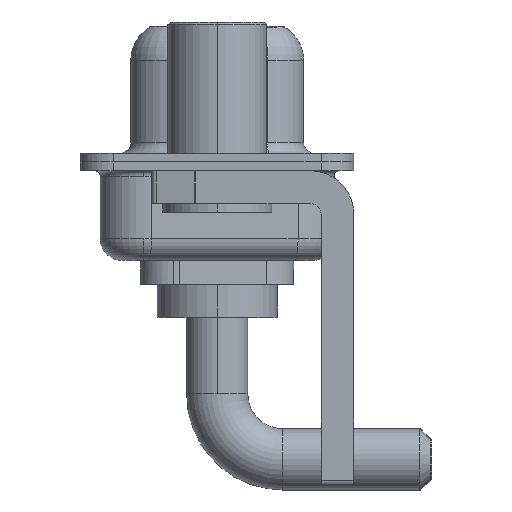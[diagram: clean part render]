
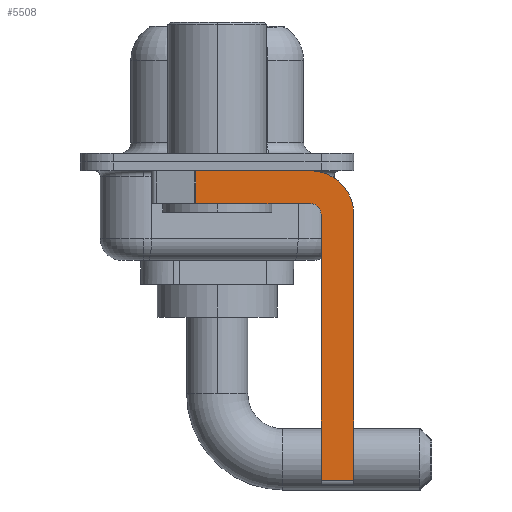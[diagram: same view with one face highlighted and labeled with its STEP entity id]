
A CAD part, left-side view. The second image highlights one B-rep face of the part: STEP entity #5508.
In plain terms, the highlighted planar face has unit normal (-1, 0, 0).
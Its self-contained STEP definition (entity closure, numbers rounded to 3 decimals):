
#677 = LINE ( 'NONE', #7979, #12336 ) ;
#777 = LINE ( 'NONE', #11700, #1538 ) ;
#812 = EDGE_CURVE ( 'NONE', #5361, #9923, #4847, .T. ) ;
#1538 = VECTOR ( 'NONE', #4550, 1000. ) ;
#1557 = AXIS2_PLACEMENT_3D ( 'NONE', #3761, #6102, #3675 ) ;
#2128 = VERTEX_POINT ( 'NONE', #10111 ) ;
#2206 = CARTESIAN_POINT ( 'NONE',  ( -2.9, 3., -0.4 ) ) ;
#2363 = CARTESIAN_POINT ( 'NONE',  ( -2.9, -4.25, -1.9 ) ) ;
#2374 = ORIENTED_EDGE ( 'NONE', *, *, #7991, .F. ) ;
#2444 = LINE ( 'NONE', #2363, #6817 ) ;
#2499 = AXIS2_PLACEMENT_3D ( 'NONE', #13245, #7312, #13542 ) ;
#2978 = VERTEX_POINT ( 'NONE', #5662 ) ;
#3033 = EDGE_CURVE ( 'NONE', #4386, #2978, #11764, .T. ) ;
#3071 = LINE ( 'NONE', #9015, #6953 ) ;
#3115 = CIRCLE ( 'NONE', #6193, 0.5 ) ;
#3116 = DIRECTION ( 'NONE',  ( -1., 0., 0. ) ) ;
#3157 = EDGE_CURVE ( 'NONE', #14407, #2128, #2444, .T. ) ;
#3183 = DIRECTION ( 'NONE',  ( 0., -1., 0. ) ) ;
#3310 = ORIENTED_EDGE ( 'NONE', *, *, #11388, .F. ) ;
#3675 = DIRECTION ( 'NONE',  ( 0., 0., -1. ) ) ;
#3761 = CARTESIAN_POINT ( 'NONE',  ( -2.9, -4.25, -2.4 ) ) ;
#3883 = CARTESIAN_POINT ( 'NONE',  ( -2.9, -4.25, -14.55 ) ) ;
#4066 = ORIENTED_EDGE ( 'NONE', *, *, #15296, .F. ) ;
#4386 = VERTEX_POINT ( 'NONE', #14305 ) ;
#4550 = DIRECTION ( 'NONE',  ( 0., 0., -1. ) ) ;
#4676 = CARTESIAN_POINT ( 'NONE',  ( -2.9, -4.25, -1.9 ) ) ;
#4727 = EDGE_LOOP ( 'NONE', ( #10317, #12907, #7708, #7586, #3310, #14551, #4066, #2374 ) ) ;
#4847 = LINE ( 'NONE', #3883, #8808 ) ;
#5361 = VERTEX_POINT ( 'NONE', #13079 ) ;
#5508 = ADVANCED_FACE ( 'NONE', ( #13474 ), #8686, .F. ) ;
#5662 = CARTESIAN_POINT ( 'NONE',  ( -2.9, -4.25, -0.4 ) ) ;
#5808 = CARTESIAN_POINT ( 'NONE',  ( -2.9, -6.25, -2.4 ) ) ;
#6102 = DIRECTION ( 'NONE',  ( 1., 0., 0. ) ) ;
#6193 = AXIS2_PLACEMENT_3D ( 'NONE', #15276, #3116, #14318 ) ;
#6817 = VECTOR ( 'NONE', #15815, 1000. ) ;
#6953 = VECTOR ( 'NONE', #15230, 1000. ) ;
#6992 = EDGE_CURVE ( 'NONE', #4386, #2128, #3071, .T. ) ;
#7120 = VERTEX_POINT ( 'NONE', #7720 ) ;
#7312 = DIRECTION ( 'NONE',  ( 1., 0., 0. ) ) ;
#7586 = ORIENTED_EDGE ( 'NONE', *, *, #9136, .F. ) ;
#7708 = ORIENTED_EDGE ( 'NONE', *, *, #3157, .F. ) ;
#7720 = CARTESIAN_POINT ( 'NONE',  ( -2.9, -4.75, -2.4 ) ) ;
#7979 = CARTESIAN_POINT ( 'NONE',  ( -2.9, -4.75, -14.8 ) ) ;
#7991 = EDGE_CURVE ( 'NONE', #2978, #8570, #12068, .T. ) ;
#8570 = VERTEX_POINT ( 'NONE', #5808 ) ;
#8686 = PLANE ( 'NONE',  #2499 ) ;
#8808 = VECTOR ( 'NONE', #14842, 1000. ) ;
#9015 = CARTESIAN_POINT ( 'NONE',  ( -2.9, 0.978, -1.9 ) ) ;
#9110 = CARTESIAN_POINT ( 'NONE',  ( -2.9, -6.25, -14.55 ) ) ;
#9136 = EDGE_CURVE ( 'NONE', #7120, #14407, #3115, .T. ) ;
#9923 = VERTEX_POINT ( 'NONE', #9110 ) ;
#10111 = CARTESIAN_POINT ( 'NONE',  ( -2.9, 0.978, -1.9 ) ) ;
#10317 = ORIENTED_EDGE ( 'NONE', *, *, #3033, .F. ) ;
#11388 = EDGE_CURVE ( 'NONE', #5361, #7120, #677, .T. ) ;
#11700 = CARTESIAN_POINT ( 'NONE',  ( -2.9, -6.25, -2.4 ) ) ;
#11764 = LINE ( 'NONE', #2206, #12184 ) ;
#12068 = CIRCLE ( 'NONE', #1557, 2. ) ;
#12184 = VECTOR ( 'NONE', #3183, 1000. ) ;
#12336 = VECTOR ( 'NONE', #15316, 1000. ) ;
#12907 = ORIENTED_EDGE ( 'NONE', *, *, #6992, .T. ) ;
#13079 = CARTESIAN_POINT ( 'NONE',  ( -2.9, -4.75, -14.55 ) ) ;
#13245 = CARTESIAN_POINT ( 'NONE',  ( -2.9, -4.25, -2.4 ) ) ;
#13474 = FACE_OUTER_BOUND ( 'NONE', #4727, .T. ) ;
#13542 = DIRECTION ( 'NONE',  ( 0., 0., -1. ) ) ;
#14305 = CARTESIAN_POINT ( 'NONE',  ( -2.9, 0.978, -0.4 ) ) ;
#14318 = DIRECTION ( 'NONE',  ( 0., 0., 1. ) ) ;
#14407 = VERTEX_POINT ( 'NONE', #4676 ) ;
#14551 = ORIENTED_EDGE ( 'NONE', *, *, #812, .T. ) ;
#14842 = DIRECTION ( 'NONE',  ( 0., -1., 0. ) ) ;
#15230 = DIRECTION ( 'NONE',  ( 0., 0., -1. ) ) ;
#15276 = CARTESIAN_POINT ( 'NONE',  ( -2.9, -4.25, -2.4 ) ) ;
#15296 = EDGE_CURVE ( 'NONE', #8570, #9923, #777, .T. ) ;
#15316 = DIRECTION ( 'NONE',  ( 0., 0., 1. ) ) ;
#15815 = DIRECTION ( 'NONE',  ( 0., 1., 0. ) ) ;
